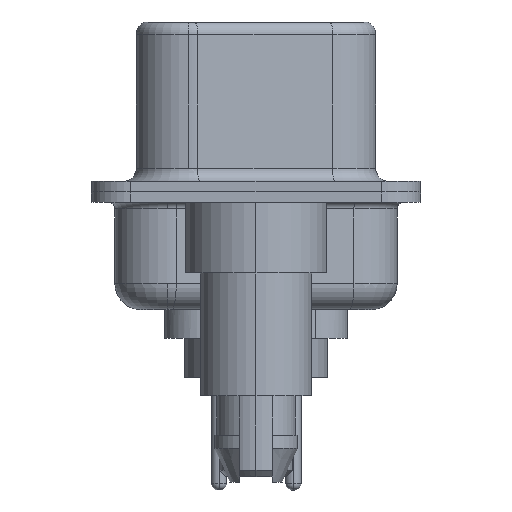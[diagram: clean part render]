
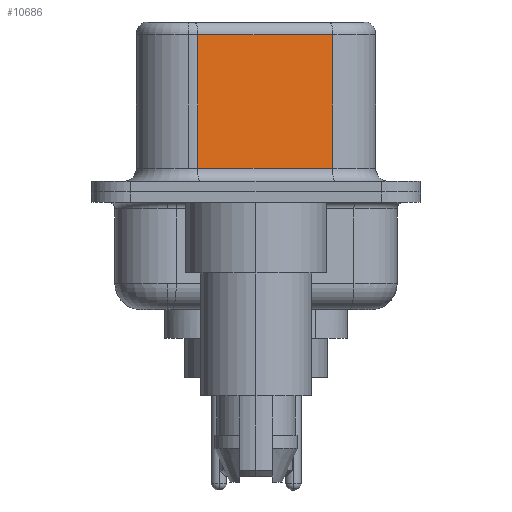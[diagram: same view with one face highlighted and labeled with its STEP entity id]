
A CAD part, left-side view. The second image highlights one B-rep face of the part: STEP entity #10686.
In plain terms, the highlighted planar face has unit normal (-0.985, -0.174, 0).
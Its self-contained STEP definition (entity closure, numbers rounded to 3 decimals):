
#1309 = CARTESIAN_POINT ( 'NONE',  ( 4.585, -2.927, 0.9 ) ) ;
#1360 = EDGE_CURVE ( 'NONE', #17812, #15008, #12938, .T. ) ;
#1820 = CARTESIAN_POINT ( 'NONE',  ( 4.585, -2.927, 6.52 ) ) ;
#2288 = CARTESIAN_POINT ( 'NONE',  ( 3.675, 2.233, 0.9 ) ) ;
#2438 = VERTEX_POINT ( 'NONE', #9597 ) ;
#3018 = FACE_OUTER_BOUND ( 'NONE', #9328, .T. ) ;
#3088 = ORIENTED_EDGE ( 'NONE', *, *, #18813, .T. ) ;
#3666 = EDGE_CURVE ( 'NONE', #18013, #2438, #18638, .T. ) ;
#4810 = PLANE ( 'NONE',  #16965 ) ;
#5744 = CARTESIAN_POINT ( 'NONE',  ( 3.675, 2.233, 6.52 ) ) ;
#6291 = DIRECTION ( 'NONE',  ( -0.174, 0.985, 0. ) ) ;
#6350 = VECTOR ( 'NONE', #10044, 1000. ) ;
#6460 = CARTESIAN_POINT ( 'NONE',  ( 4.585, -2.927, 6.02 ) ) ;
#7124 = EDGE_CURVE ( 'NONE', #17812, #2438, #17955, .T. ) ;
#9009 = VECTOR ( 'NONE', #15208, 1000. ) ;
#9328 = EDGE_LOOP ( 'NONE', ( #16116, #12105, #3088, #10868 ) ) ;
#9597 = CARTESIAN_POINT ( 'NONE',  ( 4.585, -2.927, 0.9 ) ) ;
#10037 = VECTOR ( 'NONE', #14616, 1000. ) ;
#10044 = DIRECTION ( 'NONE',  ( 0.174, -0.985, 0. ) ) ;
#10129 = CARTESIAN_POINT ( 'NONE',  ( 4.585, -2.927, 6.52 ) ) ;
#10686 = ADVANCED_FACE ( 'NONE', ( #3018 ), #4810, .F. ) ;
#10716 = VECTOR ( 'NONE', #17619, 1000. ) ;
#10868 = ORIENTED_EDGE ( 'NONE', *, *, #3666, .T. ) ;
#11175 = LINE ( 'NONE', #5744, #10716 ) ;
#12105 = ORIENTED_EDGE ( 'NONE', *, *, #1360, .T. ) ;
#12130 = CARTESIAN_POINT ( 'NONE',  ( 3.675, 2.233, 6.02 ) ) ;
#12938 = LINE ( 'NONE', #6460, #9009 ) ;
#14616 = DIRECTION ( 'NONE',  ( 0., 0., -1. ) ) ;
#15008 = VERTEX_POINT ( 'NONE', #12130 ) ;
#15179 = DIRECTION ( 'NONE',  ( 0.985, 0.174, 0. ) ) ;
#15208 = DIRECTION ( 'NONE',  ( -0.174, 0.985, 0. ) ) ;
#16116 = ORIENTED_EDGE ( 'NONE', *, *, #7124, .F. ) ;
#16965 = AXIS2_PLACEMENT_3D ( 'NONE', #1820, #15179, #6291 ) ;
#17619 = DIRECTION ( 'NONE',  ( 0., 0., -1. ) ) ;
#17812 = VERTEX_POINT ( 'NONE', #18170 ) ;
#17955 = LINE ( 'NONE', #10129, #10037 ) ;
#18013 = VERTEX_POINT ( 'NONE', #2288 ) ;
#18170 = CARTESIAN_POINT ( 'NONE',  ( 4.585, -2.927, 6.02 ) ) ;
#18638 = LINE ( 'NONE', #1309, #6350 ) ;
#18813 = EDGE_CURVE ( 'NONE', #15008, #18013, #11175, .T. ) ;
